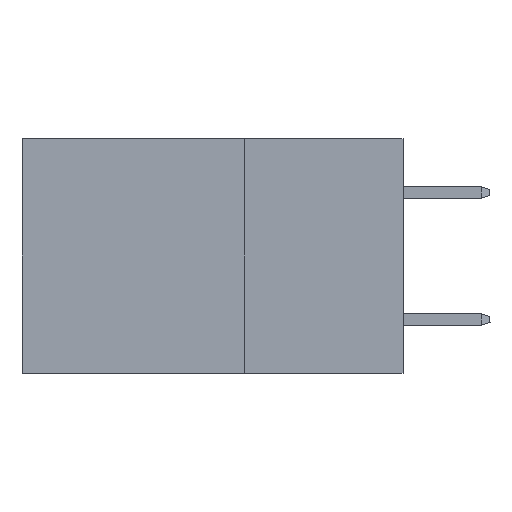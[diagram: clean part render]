
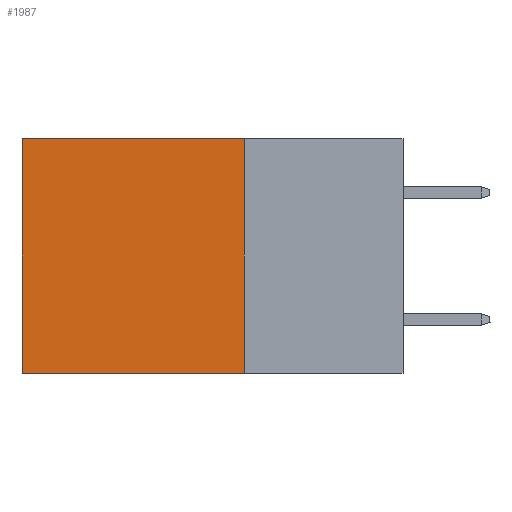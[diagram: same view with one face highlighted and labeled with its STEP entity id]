
A CAD part, left-side view. The second image highlights one B-rep face of the part: STEP entity #1987.
In plain terms, the highlighted planar face has unit normal (-1, 0, 0).
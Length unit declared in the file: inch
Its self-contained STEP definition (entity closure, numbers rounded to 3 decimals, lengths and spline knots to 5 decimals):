
#241 = ORIENTED_EDGE ( 'NONE', *, *, #13417, .T. ) ;
#560 = PLANE ( 'NONE',  #10917 ) ;
#603 = LINE ( 'NONE', #2320, #1128 ) ;
#1128 = VECTOR ( 'NONE', #16158, 39.37008 ) ;
#1251 = LINE ( 'NONE', #11053, #13929 ) ;
#1987 = ADVANCED_FACE ( 'NONE', ( #11990 ), #560, .F. ) ;
#2293 = CARTESIAN_POINT ( 'NONE',  ( 0.2875, 0.25, 0. ) ) ;
#2320 = CARTESIAN_POINT ( 'NONE',  ( 0.2875, 0.25, 0. ) ) ;
#2865 = ORIENTED_EDGE ( 'NONE', *, *, #4383, .T. ) ;
#4055 = CARTESIAN_POINT ( 'NONE',  ( 0.2875, 0.6, 0. ) ) ;
#4092 = VERTEX_POINT ( 'NONE', #2293 ) ;
#4383 = EDGE_CURVE ( 'NONE', #4699, #13246, #1251, .T. ) ;
#4699 = VERTEX_POINT ( 'NONE', #4055 ) ;
#4868 = EDGE_LOOP ( 'NONE', ( #2865, #15326, #5392, #241 ) ) ;
#5078 = DIRECTION ( 'NONE',  ( 0., 0., -1. ) ) ;
#5392 = ORIENTED_EDGE ( 'NONE', *, *, #13439, .F. ) ;
#5514 = DIRECTION ( 'NONE',  ( 0., 0., -1. ) ) ;
#9523 = CARTESIAN_POINT ( 'NONE',  ( 0.2875, 0.25, -0.37 ) ) ;
#9838 = CARTESIAN_POINT ( 'NONE',  ( 0.2875, 0.25, -0.37 ) ) ;
#10407 = VECTOR ( 'NONE', #13210, 39.37008 ) ;
#10917 = AXIS2_PLACEMENT_3D ( 'NONE', #13072, #14747, #5078 ) ;
#11053 = CARTESIAN_POINT ( 'NONE',  ( 0.2875, 0.6, 0. ) ) ;
#11352 = VERTEX_POINT ( 'NONE', #9523 ) ;
#11990 = FACE_OUTER_BOUND ( 'NONE', #4868, .T. ) ;
#12946 = CARTESIAN_POINT ( 'NONE',  ( 0.2875, 0.6, -0.37 ) ) ;
#13072 = CARTESIAN_POINT ( 'NONE',  ( 0.2875, 0.25, 0. ) ) ;
#13119 = LINE ( 'NONE', #16060, #10407 ) ;
#13210 = DIRECTION ( 'NONE',  ( 0., 0., -1. ) ) ;
#13246 = VERTEX_POINT ( 'NONE', #12946 ) ;
#13417 = EDGE_CURVE ( 'NONE', #4092, #4699, #603, .T. ) ;
#13439 = EDGE_CURVE ( 'NONE', #4092, #11352, #13119, .T. ) ;
#13731 = EDGE_CURVE ( 'NONE', #11352, #13246, #14380, .T. ) ;
#13929 = VECTOR ( 'NONE', #5514, 39.37008 ) ;
#14380 = LINE ( 'NONE', #9838, #17147 ) ;
#14747 = DIRECTION ( 'NONE',  ( 1., 0., 0. ) ) ;
#15326 = ORIENTED_EDGE ( 'NONE', *, *, #13731, .F. ) ;
#16060 = CARTESIAN_POINT ( 'NONE',  ( 0.2875, 0.25, 0. ) ) ;
#16158 = DIRECTION ( 'NONE',  ( 0., 1., 0. ) ) ;
#17140 = DIRECTION ( 'NONE',  ( 0., 1., 0. ) ) ;
#17147 = VECTOR ( 'NONE', #17140, 39.37008 ) ;
